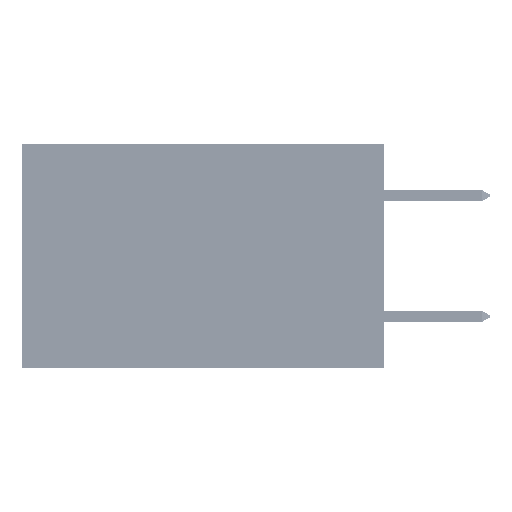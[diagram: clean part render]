
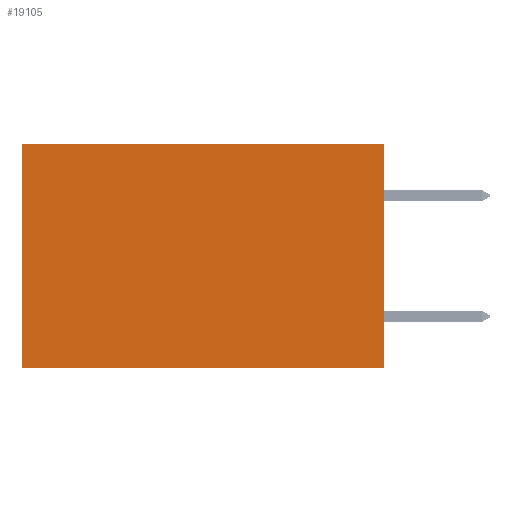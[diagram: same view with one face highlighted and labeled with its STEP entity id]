
A CAD part, left-side view. The second image highlights one B-rep face of the part: STEP entity #19105.
In plain terms, the highlighted planar face has unit normal (-1, 0, 0).
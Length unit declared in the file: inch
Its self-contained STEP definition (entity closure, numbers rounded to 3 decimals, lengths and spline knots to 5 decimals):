
#116 = EDGE_CURVE ( 'NONE', #1828, #10939, #8832, .T. ) ;
#1369 = DIRECTION ( 'NONE',  ( 0., 0., -1. ) ) ;
#1828 = VERTEX_POINT ( 'NONE', #37273 ) ;
#2246 = ORIENTED_EDGE ( 'NONE', *, *, #27228, .F. ) ;
#4494 = VERTEX_POINT ( 'NONE', #9569 ) ;
#5631 = DIRECTION ( 'NONE',  ( 0., 0., -1. ) ) ;
#6086 = CARTESIAN_POINT ( 'NONE',  ( 0.2875, 0., 0. ) ) ;
#8824 = DIRECTION ( 'NONE',  ( 0., 0., -1. ) ) ;
#8832 = LINE ( 'NONE', #10713, #17563 ) ;
#9308 = VECTOR ( 'NONE', #30896, 39.37008 ) ;
#9569 = CARTESIAN_POINT ( 'NONE',  ( 0.2875, 0.6, -0.37 ) ) ;
#10713 = CARTESIAN_POINT ( 'NONE',  ( 0.2875, 0., 0. ) ) ;
#10939 = VERTEX_POINT ( 'NONE', #15136 ) ;
#11803 = ORIENTED_EDGE ( 'NONE', *, *, #42316, .T. ) ;
#12762 = VERTEX_POINT ( 'NONE', #38568 ) ;
#13530 = CARTESIAN_POINT ( 'NONE',  ( 0.2875, 0., -0.37 ) ) ;
#15136 = CARTESIAN_POINT ( 'NONE',  ( 0.2875, 0.6, 0. ) ) ;
#17563 = VECTOR ( 'NONE', #19943, 39.37008 ) ;
#19105 = ADVANCED_FACE ( 'NONE', ( #41190 ), #40792, .F. ) ;
#19914 = DIRECTION ( 'NONE',  ( 1., 0., 0. ) ) ;
#19943 = DIRECTION ( 'NONE',  ( 0., 1., 0. ) ) ;
#20082 = LINE ( 'NONE', #22381, #31558 ) ;
#20223 = ORIENTED_EDGE ( 'NONE', *, *, #44861, .F. ) ;
#22381 = CARTESIAN_POINT ( 'NONE',  ( 0.2875, 0., 0. ) ) ;
#23376 = EDGE_LOOP ( 'NONE', ( #11803, #20223, #2246, #39690 ) ) ;
#27228 = EDGE_CURVE ( 'NONE', #1828, #12762, #20082, .T. ) ;
#29317 = CARTESIAN_POINT ( 'NONE',  ( 0.2875, 0.6, 0. ) ) ;
#30896 = DIRECTION ( 'NONE',  ( 0., 1., 0. ) ) ;
#31558 = VECTOR ( 'NONE', #8824, 39.37008 ) ;
#33445 = VECTOR ( 'NONE', #1369, 39.37008 ) ;
#37273 = CARTESIAN_POINT ( 'NONE',  ( 0.2875, 0., 0. ) ) ;
#38568 = CARTESIAN_POINT ( 'NONE',  ( 0.2875, 0., -0.37 ) ) ;
#38892 = LINE ( 'NONE', #29317, #33445 ) ;
#39690 = ORIENTED_EDGE ( 'NONE', *, *, #116, .T. ) ;
#40792 = PLANE ( 'NONE',  #44789 ) ;
#40917 = LINE ( 'NONE', #13530, #9308 ) ;
#41190 = FACE_OUTER_BOUND ( 'NONE', #23376, .T. ) ;
#42316 = EDGE_CURVE ( 'NONE', #10939, #4494, #38892, .T. ) ;
#44789 = AXIS2_PLACEMENT_3D ( 'NONE', #6086, #19914, #5631 ) ;
#44861 = EDGE_CURVE ( 'NONE', #12762, #4494, #40917, .T. ) ;
